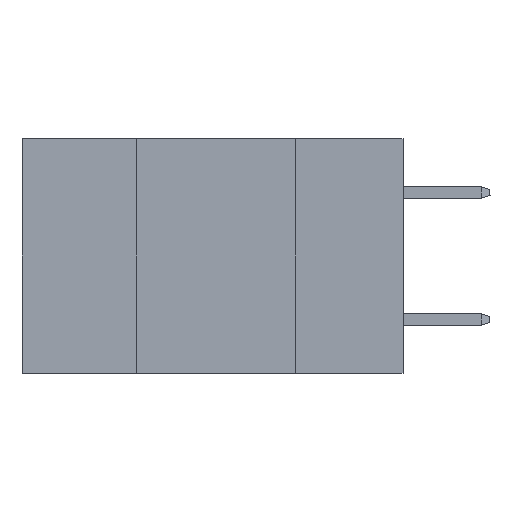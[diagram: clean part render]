
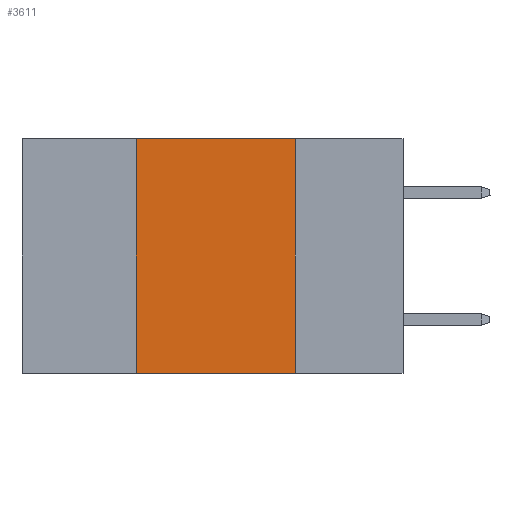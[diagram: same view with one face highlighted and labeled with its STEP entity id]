
A CAD part, left-side view. The second image highlights one B-rep face of the part: STEP entity #3611.
In plain terms, the highlighted planar face has unit normal (-1, 0, 0).
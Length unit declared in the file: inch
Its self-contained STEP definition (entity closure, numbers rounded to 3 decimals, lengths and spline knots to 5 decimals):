
#1057 = ORIENTED_EDGE ( 'NONE', *, *, #23510, .T. ) ;
#1238 = VECTOR ( 'NONE', #37646, 39.37008 ) ;
#2740 = CARTESIAN_POINT ( 'NONE',  ( 0., 0.17, -0.37 ) ) ;
#3611 = ADVANCED_FACE ( 'NONE', ( #5302 ), #7996, .F. ) ;
#3715 = VERTEX_POINT ( 'NONE', #21059 ) ;
#5302 = FACE_OUTER_BOUND ( 'NONE', #22654, .T. ) ;
#6227 = CARTESIAN_POINT ( 'NONE',  ( 0., 0.42, -0.37 ) ) ;
#7408 = ORIENTED_EDGE ( 'NONE', *, *, #23556, .F. ) ;
#7794 = EDGE_CURVE ( 'NONE', #26515, #37429, #20931, .T. ) ;
#7955 = VECTOR ( 'NONE', #23634, 39.37008 ) ;
#7996 = PLANE ( 'NONE',  #40578 ) ;
#8698 = EDGE_CURVE ( 'NONE', #20450, #3715, #25081, .T. ) ;
#9013 = ORIENTED_EDGE ( 'NONE', *, *, #8698, .F. ) ;
#11591 = CARTESIAN_POINT ( 'NONE',  ( 0., 0.17, 0. ) ) ;
#11646 = CARTESIAN_POINT ( 'NONE',  ( 0., 0.42, 0. ) ) ;
#13662 = LINE ( 'NONE', #39487, #22490 ) ;
#17952 = CARTESIAN_POINT ( 'NONE',  ( 0., 0.6, 0. ) ) ;
#20450 = VERTEX_POINT ( 'NONE', #6227 ) ;
#20537 = DIRECTION ( 'NONE',  ( 0., -1., 0. ) ) ;
#20931 = LINE ( 'NONE', #11591, #22370 ) ;
#21059 = CARTESIAN_POINT ( 'NONE',  ( 0., 0.42, 0. ) ) ;
#22370 = VECTOR ( 'NONE', #28494, 39.37008 ) ;
#22490 = VECTOR ( 'NONE', #20537, 39.37008 ) ;
#22654 = EDGE_LOOP ( 'NONE', ( #30199, #7408, #9013, #1057 ) ) ;
#23510 = EDGE_CURVE ( 'NONE', #20450, #37429, #13662, .T. ) ;
#23556 = EDGE_CURVE ( 'NONE', #3715, #26515, #35561, .T. ) ;
#23634 = DIRECTION ( 'NONE',  ( 0., -1., 0. ) ) ;
#23969 = DIRECTION ( 'NONE',  ( 1., 0., 0. ) ) ;
#25081 = LINE ( 'NONE', #11646, #1238 ) ;
#26515 = VERTEX_POINT ( 'NONE', #32934 ) ;
#28494 = DIRECTION ( 'NONE',  ( 0., 0., -1. ) ) ;
#29616 = CARTESIAN_POINT ( 'NONE',  ( 0., 0.6, 0. ) ) ;
#30199 = ORIENTED_EDGE ( 'NONE', *, *, #7794, .F. ) ;
#30573 = DIRECTION ( 'NONE',  ( 0., 0., -1. ) ) ;
#32934 = CARTESIAN_POINT ( 'NONE',  ( 0., 0.17, 0. ) ) ;
#35561 = LINE ( 'NONE', #29616, #7955 ) ;
#37429 = VERTEX_POINT ( 'NONE', #2740 ) ;
#37646 = DIRECTION ( 'NONE',  ( 0., 0., 1. ) ) ;
#39487 = CARTESIAN_POINT ( 'NONE',  ( 0., 0.6, -0.37 ) ) ;
#40578 = AXIS2_PLACEMENT_3D ( 'NONE', #17952, #23969, #30573 ) ;
